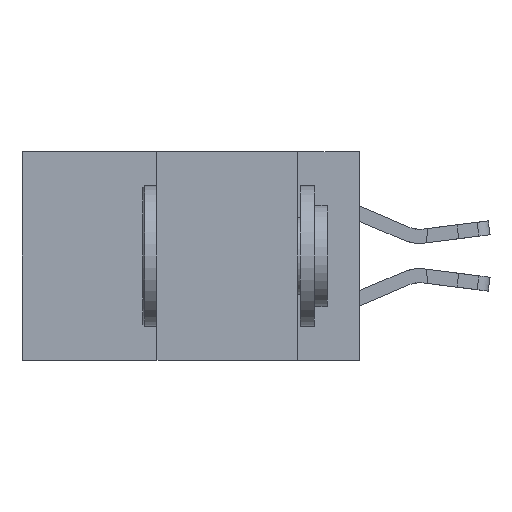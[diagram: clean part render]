
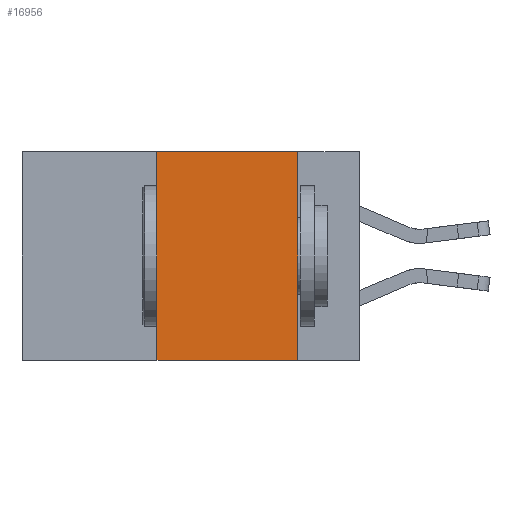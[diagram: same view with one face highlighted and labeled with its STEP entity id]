
A CAD part, left-side view. The second image highlights one B-rep face of the part: STEP entity #16956.
In plain terms, the highlighted planar face has unit normal (-1, 0, 0).
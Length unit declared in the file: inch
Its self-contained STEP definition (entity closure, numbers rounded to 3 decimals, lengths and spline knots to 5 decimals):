
#1001 = VERTEX_POINT ( 'NONE', #6479 ) ;
#2561 = VECTOR ( 'NONE', #3735, 39.37008 ) ;
#2886 = VERTEX_POINT ( 'NONE', #3292 ) ;
#3111 = CARTESIAN_POINT ( 'NONE',  ( 0., 0.6, 0. ) ) ;
#3292 = CARTESIAN_POINT ( 'NONE',  ( 0., 0.36, -0.37 ) ) ;
#3298 = DIRECTION ( 'NONE',  ( 0., -1., 0. ) ) ;
#3494 = CARTESIAN_POINT ( 'NONE',  ( 0., 0.11, 0. ) ) ;
#3735 = DIRECTION ( 'NONE',  ( 0., 0., -1. ) ) ;
#3845 = FACE_OUTER_BOUND ( 'NONE', #5328, .T. ) ;
#4107 = AXIS2_PLACEMENT_3D ( 'NONE', #3111, #4553, #7467 ) ;
#4129 = VECTOR ( 'NONE', #9499, 39.37008 ) ;
#4553 = DIRECTION ( 'NONE',  ( 1., 0., 0. ) ) ;
#5257 = CARTESIAN_POINT ( 'NONE',  ( 0., 0.11, 0. ) ) ;
#5328 = EDGE_LOOP ( 'NONE', ( #9809, #7986, #17649, #12466 ) ) ;
#5892 = PLANE ( 'NONE',  #4107 ) ;
#6035 = VECTOR ( 'NONE', #8013, 39.37008 ) ;
#6479 = CARTESIAN_POINT ( 'NONE',  ( 0., 0.36, 0. ) ) ;
#7168 = LINE ( 'NONE', #9314, #6035 ) ;
#7467 = DIRECTION ( 'NONE',  ( 0., 0., -1. ) ) ;
#7934 = EDGE_CURVE ( 'NONE', #2886, #1001, #7168, .T. ) ;
#7986 = ORIENTED_EDGE ( 'NONE', *, *, #11770, .F. ) ;
#8013 = DIRECTION ( 'NONE',  ( 0., 0., 1. ) ) ;
#9121 = LINE ( 'NONE', #10448, #9822 ) ;
#9314 = CARTESIAN_POINT ( 'NONE',  ( 0., 0.36, 0. ) ) ;
#9315 = CARTESIAN_POINT ( 'NONE',  ( 0., 0.6, 0. ) ) ;
#9499 = DIRECTION ( 'NONE',  ( 0., -1., 0. ) ) ;
#9809 = ORIENTED_EDGE ( 'NONE', *, *, #11790, .F. ) ;
#9822 = VECTOR ( 'NONE', #3298, 39.37008 ) ;
#10288 = VERTEX_POINT ( 'NONE', #13404 ) ;
#10294 = EDGE_CURVE ( 'NONE', #2886, #10288, #9121, .T. ) ;
#10448 = CARTESIAN_POINT ( 'NONE',  ( 0., 0.6, -0.37 ) ) ;
#11770 = EDGE_CURVE ( 'NONE', #1001, #17289, #14236, .T. ) ;
#11790 = EDGE_CURVE ( 'NONE', #17289, #10288, #14016, .T. ) ;
#12466 = ORIENTED_EDGE ( 'NONE', *, *, #10294, .T. ) ;
#13404 = CARTESIAN_POINT ( 'NONE',  ( 0., 0.11, -0.37 ) ) ;
#14016 = LINE ( 'NONE', #5257, #2561 ) ;
#14236 = LINE ( 'NONE', #9315, #4129 ) ;
#16956 = ADVANCED_FACE ( 'NONE', ( #3845 ), #5892, .F. ) ;
#17289 = VERTEX_POINT ( 'NONE', #3494 ) ;
#17649 = ORIENTED_EDGE ( 'NONE', *, *, #7934, .F. ) ;
